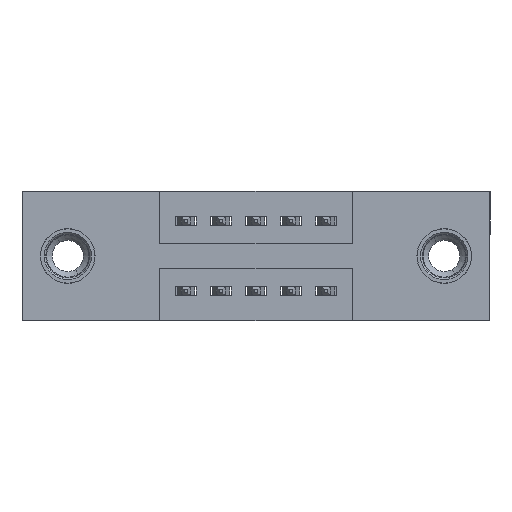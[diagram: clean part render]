
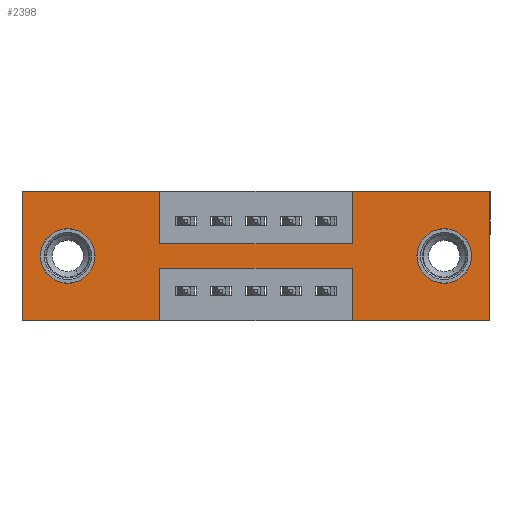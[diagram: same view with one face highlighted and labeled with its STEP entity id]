
A CAD part, front view. The second image highlights one B-rep face of the part: STEP entity #2398.
In plain terms, the highlighted planar face has unit normal (0, -1, 0).
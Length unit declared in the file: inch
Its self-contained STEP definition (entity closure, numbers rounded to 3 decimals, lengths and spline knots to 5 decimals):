
#3 = VECTOR ( 'NONE', #5656, 39.37008 ) ;
#298 = EDGE_CURVE ( 'NONE', #8269, #1930, #13032, .T. ) ;
#320 = EDGE_CURVE ( 'NONE', #5351, #1937, #10388, .T. ) ;
#427 = ORIENTED_EDGE ( 'NONE', *, *, #11081, .F. ) ;
#658 = VERTEX_POINT ( 'NONE', #9378 ) ;
#708 = LINE ( 'NONE', #12179, #3587 ) ;
#736 = CIRCLE ( 'NONE', #2001, 0.078 ) ;
#880 = FACE_BOUND ( 'NONE', #7388, .T. ) ;
#961 = DIRECTION ( 'NONE',  ( 0., 1., 0. ) ) ;
#1049 = LINE ( 'NONE', #10603, #12238 ) ;
#1059 = DIRECTION ( 'NONE',  ( 0., 1., 0. ) ) ;
#1066 = CARTESIAN_POINT ( 'NONE',  ( 0.13, 0., -0.107 ) ) ;
#1278 = DIRECTION ( 'NONE',  ( -1., 0., 0. ) ) ;
#1337 = VERTEX_POINT ( 'NONE', #7494 ) ;
#1367 = ORIENTED_EDGE ( 'NONE', *, *, #9096, .F. ) ;
#1770 = DIRECTION ( 'NONE',  ( 0., 1., 0. ) ) ;
#1895 = LINE ( 'NONE', #7610, #12370 ) ;
#1926 = CARTESIAN_POINT ( 'NONE',  ( 1.205, 0., -0.185 ) ) ;
#1930 = VERTEX_POINT ( 'NONE', #10601 ) ;
#1932 = EDGE_CURVE ( 'NONE', #6257, #5351, #2888, .T. ) ;
#1937 = VERTEX_POINT ( 'NONE', #11413 ) ;
#2001 = AXIS2_PLACEMENT_3D ( 'NONE', #7468, #1059, #8520 ) ;
#2025 = DIRECTION ( 'NONE',  ( 0., 0., 1. ) ) ;
#2398 = ADVANCED_FACE ( 'NONE', ( #880, #6605, #11785 ), #2751, .T. ) ;
#2426 = CARTESIAN_POINT ( 'NONE',  ( 0.3925, 0., 0. ) ) ;
#2427 = VERTEX_POINT ( 'NONE', #6776 ) ;
#2516 = ORIENTED_EDGE ( 'NONE', *, *, #2613, .F. ) ;
#2544 = EDGE_CURVE ( 'NONE', #2607, #8405, #10196, .T. ) ;
#2607 = VERTEX_POINT ( 'NONE', #1066 ) ;
#2613 = EDGE_CURVE ( 'NONE', #1930, #3605, #1049, .T. ) ;
#2677 = ORIENTED_EDGE ( 'NONE', *, *, #1932, .F. ) ;
#2751 = PLANE ( 'NONE',  #7566 ) ;
#2888 = LINE ( 'NONE', #7222, #13599 ) ;
#2976 = DIRECTION ( 'NONE',  ( 0., 0., -1. ) ) ;
#3175 = VECTOR ( 'NONE', #5150, 39.37008 ) ;
#3176 = CARTESIAN_POINT ( 'NONE',  ( 0.3925, 0., -0.37 ) ) ;
#3587 = VECTOR ( 'NONE', #4886, 39.37008 ) ;
#3605 = VERTEX_POINT ( 'NONE', #6172 ) ;
#3724 = VERTEX_POINT ( 'NONE', #8487 ) ;
#3733 = CARTESIAN_POINT ( 'NONE',  ( 0., 0., -0.37 ) ) ;
#3796 = VECTOR ( 'NONE', #1278, 39.37008 ) ;
#3797 = DIRECTION ( 'NONE',  ( 0., -1., 0. ) ) ;
#3931 = EDGE_CURVE ( 'NONE', #1337, #8269, #5862, .T. ) ;
#3969 = DIRECTION ( 'NONE',  ( 1., 0., 0. ) ) ;
#4054 = CARTESIAN_POINT ( 'NONE',  ( 0.3925, 0., 0. ) ) ;
#4159 = CARTESIAN_POINT ( 'NONE',  ( 0., 0., 0. ) ) ;
#4224 = VECTOR ( 'NONE', #2025, 39.37008 ) ;
#4351 = ORIENTED_EDGE ( 'NONE', *, *, #9053, .T. ) ;
#4435 = CARTESIAN_POINT ( 'NONE',  ( 0.3925, 0., -0.22 ) ) ;
#4768 = VECTOR ( 'NONE', #6892, 39.37008 ) ;
#4886 = DIRECTION ( 'NONE',  ( -1., 0., 0. ) ) ;
#4984 = VECTOR ( 'NONE', #3969, 39.37008 ) ;
#5031 = CARTESIAN_POINT ( 'NONE',  ( 1.205, 0., -0.263 ) ) ;
#5129 = AXIS2_PLACEMENT_3D ( 'NONE', #1926, #9355, #2976 ) ;
#5150 = DIRECTION ( 'NONE',  ( 0., 0., 1. ) ) ;
#5261 = DIRECTION ( 'NONE',  ( 1., 0., 0. ) ) ;
#5351 = VERTEX_POINT ( 'NONE', #4054 ) ;
#5624 = VERTEX_POINT ( 'NONE', #6043 ) ;
#5656 = DIRECTION ( 'NONE',  ( 0., 0., 1. ) ) ;
#5862 = LINE ( 'NONE', #11903, #3 ) ;
#5909 = ORIENTED_EDGE ( 'NONE', *, *, #9151, .T. ) ;
#6043 = CARTESIAN_POINT ( 'NONE',  ( 0.3925, 0., -0.37 ) ) ;
#6172 = CARTESIAN_POINT ( 'NONE',  ( 1.335, 0., -0.37 ) ) ;
#6218 = EDGE_LOOP ( 'NONE', ( #12583, #8810, #7945, #7609, #2516, #13202, #8803, #1367, #10286, #2677, #12857, #427 ) ) ;
#6257 = VERTEX_POINT ( 'NONE', #13310 ) ;
#6605 = FACE_BOUND ( 'NONE', #9869, .T. ) ;
#6776 = CARTESIAN_POINT ( 'NONE',  ( 0., 0., -0.37 ) ) ;
#6867 = DIRECTION ( 'NONE',  ( 0., 0., -1. ) ) ;
#6892 = DIRECTION ( 'NONE',  ( 1., 0., 0. ) ) ;
#6993 = EDGE_CURVE ( 'NONE', #8405, #2607, #736, .T. ) ;
#7222 = CARTESIAN_POINT ( 'NONE',  ( 0., 0., 0. ) ) ;
#7285 = VECTOR ( 'NONE', #12021, 39.37008 ) ;
#7388 = EDGE_LOOP ( 'NONE', ( #4351, #5909 ) ) ;
#7417 = LINE ( 'NONE', #4159, #4224 ) ;
#7468 = CARTESIAN_POINT ( 'NONE',  ( 0.13, 0., -0.185 ) ) ;
#7494 = CARTESIAN_POINT ( 'NONE',  ( 0.9425, 0., -0.15 ) ) ;
#7566 = AXIS2_PLACEMENT_3D ( 'NONE', #3733, #3797, #6867 ) ;
#7587 = EDGE_CURVE ( 'NONE', #8475, #658, #8523, .T. ) ;
#7609 = ORIENTED_EDGE ( 'NONE', *, *, #13328, .F. ) ;
#7610 = CARTESIAN_POINT ( 'NONE',  ( 0., 0., -0.37 ) ) ;
#7659 = CARTESIAN_POINT ( 'NONE',  ( 0.3925, 0., -0.22 ) ) ;
#7945 = ORIENTED_EDGE ( 'NONE', *, *, #7587, .F. ) ;
#8157 = CARTESIAN_POINT ( 'NONE',  ( 1.205, 0., -0.185 ) ) ;
#8269 = VERTEX_POINT ( 'NONE', #12972 ) ;
#8402 = LINE ( 'NONE', #3176, #10839 ) ;
#8405 = VERTEX_POINT ( 'NONE', #9142 ) ;
#8430 = DIRECTION ( 'NONE',  ( 0., 0., 1. ) ) ;
#8441 = LINE ( 'NONE', #7659, #3796 ) ;
#8475 = VERTEX_POINT ( 'NONE', #12279 ) ;
#8487 = CARTESIAN_POINT ( 'NONE',  ( 1.205, 0., -0.107 ) ) ;
#8520 = DIRECTION ( 'NONE',  ( 0., 0., 1. ) ) ;
#8523 = LINE ( 'NONE', #12456, #3175 ) ;
#8674 = DIRECTION ( 'NONE',  ( -1., 0., 0. ) ) ;
#8803 = ORIENTED_EDGE ( 'NONE', *, *, #3931, .F. ) ;
#8810 = ORIENTED_EDGE ( 'NONE', *, *, #10455, .F. ) ;
#8904 = ORIENTED_EDGE ( 'NONE', *, *, #6993, .T. ) ;
#9053 = EDGE_CURVE ( 'NONE', #3724, #9107, #13529, .T. ) ;
#9096 = EDGE_CURVE ( 'NONE', #1937, #1337, #10274, .T. ) ;
#9107 = VERTEX_POINT ( 'NONE', #5031 ) ;
#9142 = CARTESIAN_POINT ( 'NONE',  ( 0.13, 0., -0.263 ) ) ;
#9151 = EDGE_CURVE ( 'NONE', #9107, #3724, #12620, .T. ) ;
#9223 = DIRECTION ( 'NONE',  ( 0., 0., -1. ) ) ;
#9355 = DIRECTION ( 'NONE',  ( 0., 1., 0. ) ) ;
#9378 = CARTESIAN_POINT ( 'NONE',  ( 0.9425, 0., -0.22 ) ) ;
#9869 = EDGE_LOOP ( 'NONE', ( #12359, #8904 ) ) ;
#10169 = CARTESIAN_POINT ( 'NONE',  ( 0.13, 0., -0.185 ) ) ;
#10196 = CIRCLE ( 'NONE', #13680, 0.078 ) ;
#10274 = LINE ( 'NONE', #10297, #4984 ) ;
#10286 = ORIENTED_EDGE ( 'NONE', *, *, #320, .F. ) ;
#10297 = CARTESIAN_POINT ( 'NONE',  ( 0.3925, 0., -0.15 ) ) ;
#10388 = LINE ( 'NONE', #2426, #7285 ) ;
#10455 = EDGE_CURVE ( 'NONE', #658, #10854, #8441, .T. ) ;
#10575 = DIRECTION ( 'NONE',  ( 0., 0., -1. ) ) ;
#10601 = CARTESIAN_POINT ( 'NONE',  ( 1.335, 0., 0. ) ) ;
#10603 = CARTESIAN_POINT ( 'NONE',  ( 1.335, 0., 0. ) ) ;
#10839 = VECTOR ( 'NONE', #10575, 39.37008 ) ;
#10854 = VERTEX_POINT ( 'NONE', #4435 ) ;
#11081 = EDGE_CURVE ( 'NONE', #5624, #2427, #708, .T. ) ;
#11413 = CARTESIAN_POINT ( 'NONE',  ( 0.3925, 0., -0.15 ) ) ;
#11634 = DIRECTION ( 'NONE',  ( 0., 0., -1. ) ) ;
#11785 = FACE_OUTER_BOUND ( 'NONE', #6218, .T. ) ;
#11891 = EDGE_CURVE ( 'NONE', #10854, #5624, #8402, .T. ) ;
#11903 = CARTESIAN_POINT ( 'NONE',  ( 0.9425, 0., 0. ) ) ;
#12021 = DIRECTION ( 'NONE',  ( 0., 0., -1. ) ) ;
#12179 = CARTESIAN_POINT ( 'NONE',  ( 0., 0., -0.37 ) ) ;
#12238 = VECTOR ( 'NONE', #11634, 39.37008 ) ;
#12279 = CARTESIAN_POINT ( 'NONE',  ( 0.9425, 0., -0.37 ) ) ;
#12359 = ORIENTED_EDGE ( 'NONE', *, *, #2544, .T. ) ;
#12370 = VECTOR ( 'NONE', #8674, 39.37008 ) ;
#12406 = EDGE_CURVE ( 'NONE', #2427, #6257, #7417, .T. ) ;
#12456 = CARTESIAN_POINT ( 'NONE',  ( 0.9425, 0., -0.37 ) ) ;
#12583 = ORIENTED_EDGE ( 'NONE', *, *, #11891, .F. ) ;
#12620 = CIRCLE ( 'NONE', #5129, 0.078 ) ;
#12857 = ORIENTED_EDGE ( 'NONE', *, *, #12406, .F. ) ;
#12972 = CARTESIAN_POINT ( 'NONE',  ( 0.9425, 0., 0. ) ) ;
#13032 = LINE ( 'NONE', #13301, #4768 ) ;
#13202 = ORIENTED_EDGE ( 'NONE', *, *, #298, .F. ) ;
#13301 = CARTESIAN_POINT ( 'NONE',  ( 0., 0., 0. ) ) ;
#13310 = CARTESIAN_POINT ( 'NONE',  ( 0., 0., 0. ) ) ;
#13328 = EDGE_CURVE ( 'NONE', #3605, #8475, #1895, .T. ) ;
#13529 = CIRCLE ( 'NONE', #13665, 0.078 ) ;
#13599 = VECTOR ( 'NONE', #5261, 39.37008 ) ;
#13665 = AXIS2_PLACEMENT_3D ( 'NONE', #8157, #1770, #9223 ) ;
#13680 = AXIS2_PLACEMENT_3D ( 'NONE', #10169, #961, #8430 ) ;
